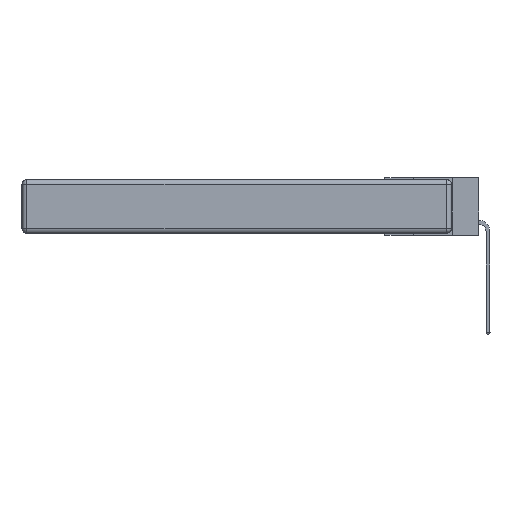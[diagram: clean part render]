
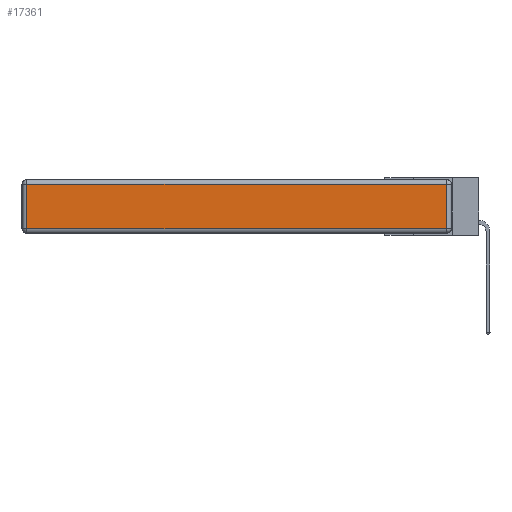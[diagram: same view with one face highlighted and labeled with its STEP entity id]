
A CAD part, left-side view. The second image highlights one B-rep face of the part: STEP entity #17361.
In plain terms, the highlighted planar face has unit normal (-1, 0, 0).
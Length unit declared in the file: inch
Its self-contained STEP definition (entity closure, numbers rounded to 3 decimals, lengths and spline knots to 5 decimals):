
#900 = VECTOR ( 'NONE', #20917, 39.37008 ) ;
#1467 = EDGE_CURVE ( 'NONE', #19733, #13556, #6269, .T. ) ;
#1908 = VECTOR ( 'NONE', #10407, 39.37008 ) ;
#2342 = ORIENTED_EDGE ( 'NONE', *, *, #17291, .T. ) ;
#2468 = ORIENTED_EDGE ( 'NONE', *, *, #30616, .T. ) ;
#3016 = LINE ( 'NONE', #10927, #18943 ) ;
#3051 = PLANE ( 'NONE',  #3914 ) ;
#3182 = CARTESIAN_POINT ( 'NONE',  ( 0., 0.03, -0.03 ) ) ;
#3914 = AXIS2_PLACEMENT_3D ( 'NONE', #5583, #15836, #25961 ) ;
#5070 = CARTESIAN_POINT ( 'NONE',  ( 0., 2.75, -0.03 ) ) ;
#5583 = CARTESIAN_POINT ( 'NONE',  ( 0., 0., -0.343 ) ) ;
#6269 = LINE ( 'NONE', #5070, #1908 ) ;
#7751 = EDGE_LOOP ( 'NONE', ( #2342, #2468, #31837, #23867 ) ) ;
#9835 = CARTESIAN_POINT ( 'NONE',  ( 0., 0., -0.313 ) ) ;
#10407 = DIRECTION ( 'NONE',  ( 0., 1., 0. ) ) ;
#10927 = CARTESIAN_POINT ( 'NONE',  ( 0., 0.03, -0.343 ) ) ;
#11771 = CARTESIAN_POINT ( 'NONE',  ( 0., 0.03, -0.313 ) ) ;
#11841 = FACE_OUTER_BOUND ( 'NONE', #7751, .T. ) ;
#13542 = EDGE_CURVE ( 'NONE', #13556, #20685, #22357, .T. ) ;
#13556 = VERTEX_POINT ( 'NONE', #26031 ) ;
#14488 = CARTESIAN_POINT ( 'NONE',  ( 0., 2.72, -0.313 ) ) ;
#15686 = CARTESIAN_POINT ( 'NONE',  ( 0., 2.72, -0.343 ) ) ;
#15836 = DIRECTION ( 'NONE',  ( -1., 0., 0. ) ) ;
#17291 = EDGE_CURVE ( 'NONE', #20685, #20144, #20002, .T. ) ;
#17361 = ADVANCED_FACE ( 'NONE', ( #11841 ), #3051, .T. ) ;
#18488 = DIRECTION ( 'NONE',  ( 0., 0., 1. ) ) ;
#18943 = VECTOR ( 'NONE', #18488, 39.37008 ) ;
#19733 = VERTEX_POINT ( 'NONE', #3182 ) ;
#20002 = LINE ( 'NONE', #9835, #30356 ) ;
#20144 = VERTEX_POINT ( 'NONE', #11771 ) ;
#20685 = VERTEX_POINT ( 'NONE', #14488 ) ;
#20917 = DIRECTION ( 'NONE',  ( 0., 0., -1. ) ) ;
#22357 = LINE ( 'NONE', #15686, #900 ) ;
#23867 = ORIENTED_EDGE ( 'NONE', *, *, #13542, .T. ) ;
#25961 = DIRECTION ( 'NONE',  ( 0., 0., 1. ) ) ;
#26031 = CARTESIAN_POINT ( 'NONE',  ( 0., 2.72, -0.03 ) ) ;
#30356 = VECTOR ( 'NONE', #32993, 39.37008 ) ;
#30616 = EDGE_CURVE ( 'NONE', #20144, #19733, #3016, .T. ) ;
#31837 = ORIENTED_EDGE ( 'NONE', *, *, #1467, .T. ) ;
#32993 = DIRECTION ( 'NONE',  ( 0., -1., 0. ) ) ;
